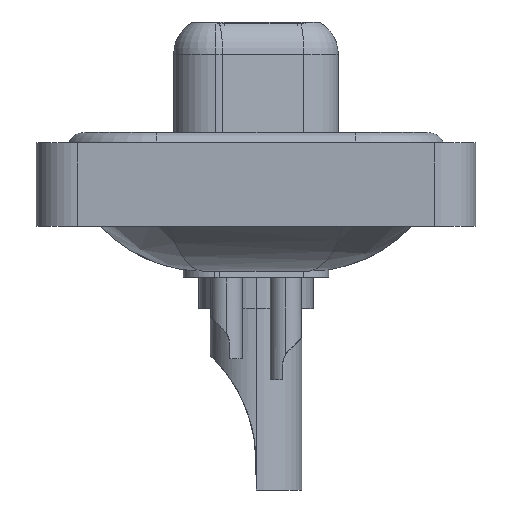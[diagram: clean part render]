
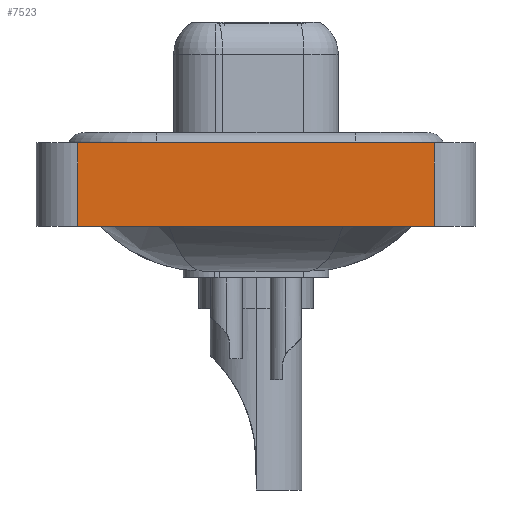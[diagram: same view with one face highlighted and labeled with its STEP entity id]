
A CAD part, left-side view. The second image highlights one B-rep face of the part: STEP entity #7523.
In plain terms, the highlighted planar face has unit normal (-1, 0, 0).
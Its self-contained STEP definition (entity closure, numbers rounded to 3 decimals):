
#382 = DIRECTION ( 'NONE',  ( 0., 0., 1. ) ) ;
#435 = LINE ( 'NONE', #18893, #10427 ) ;
#1599 = CARTESIAN_POINT ( 'NONE',  ( -7.25, -8.55, -3.6 ) ) ;
#1795 = PLANE ( 'NONE',  #18159 ) ;
#2160 = CARTESIAN_POINT ( 'NONE',  ( -7.25, -8.55, -3.6 ) ) ;
#2779 = LINE ( 'NONE', #16801, #6432 ) ;
#3050 = VERTEX_POINT ( 'NONE', #10101 ) ;
#3213 = ORIENTED_EDGE ( 'NONE', *, *, #16454, .T. ) ;
#3561 = EDGE_CURVE ( 'NONE', #3050, #8989, #4937, .T. ) ;
#3582 = ORIENTED_EDGE ( 'NONE', *, *, #13383, .T. ) ;
#4471 = EDGE_CURVE ( 'NONE', #8989, #13758, #435, .T. ) ;
#4937 = LINE ( 'NONE', #8063, #12819 ) ;
#5184 = LINE ( 'NONE', #2160, #9350 ) ;
#5292 = DIRECTION ( 'NONE',  ( 0., -1., 0. ) ) ;
#5922 = DIRECTION ( 'NONE',  ( 0., 0., 1. ) ) ;
#5972 = ORIENTED_EDGE ( 'NONE', *, *, #4471, .F. ) ;
#5994 = CARTESIAN_POINT ( 'NONE',  ( -7.25, -8.55, 0.4 ) ) ;
#6253 = DIRECTION ( 'NONE',  ( 0., 0., 1. ) ) ;
#6432 = VECTOR ( 'NONE', #5922, 1000. ) ;
#7523 = ADVANCED_FACE ( 'NONE', ( #9180 ), #1795, .T. ) ;
#8063 = CARTESIAN_POINT ( 'NONE',  ( -7.25, 8.55, -3.6 ) ) ;
#8467 = CARTESIAN_POINT ( 'NONE',  ( -7.25, -8.55, -3.6 ) ) ;
#8989 = VERTEX_POINT ( 'NONE', #14348 ) ;
#9180 = FACE_OUTER_BOUND ( 'NONE', #16797, .T. ) ;
#9350 = VECTOR ( 'NONE', #9838, 1000. ) ;
#9838 = DIRECTION ( 'NONE',  ( 0., -1., 0. ) ) ;
#9940 = VERTEX_POINT ( 'NONE', #8467 ) ;
#10101 = CARTESIAN_POINT ( 'NONE',  ( -7.25, 8.55, -3.6 ) ) ;
#10427 = VECTOR ( 'NONE', #5292, 1000. ) ;
#12819 = VECTOR ( 'NONE', #382, 1000. ) ;
#13383 = EDGE_CURVE ( 'NONE', #9940, #13758, #2779, .T. ) ;
#13758 = VERTEX_POINT ( 'NONE', #5994 ) ;
#14217 = DIRECTION ( 'NONE',  ( -1., 0., 0. ) ) ;
#14348 = CARTESIAN_POINT ( 'NONE',  ( -7.25, 8.55, 0.4 ) ) ;
#16218 = ORIENTED_EDGE ( 'NONE', *, *, #3561, .F. ) ;
#16454 = EDGE_CURVE ( 'NONE', #3050, #9940, #5184, .T. ) ;
#16797 = EDGE_LOOP ( 'NONE', ( #3582, #5972, #16218, #3213 ) ) ;
#16801 = CARTESIAN_POINT ( 'NONE',  ( -7.25, -8.55, -3.6 ) ) ;
#18159 = AXIS2_PLACEMENT_3D ( 'NONE', #1599, #14217, #6253 ) ;
#18893 = CARTESIAN_POINT ( 'NONE',  ( -7.25, -8.55, 0.4 ) ) ;
